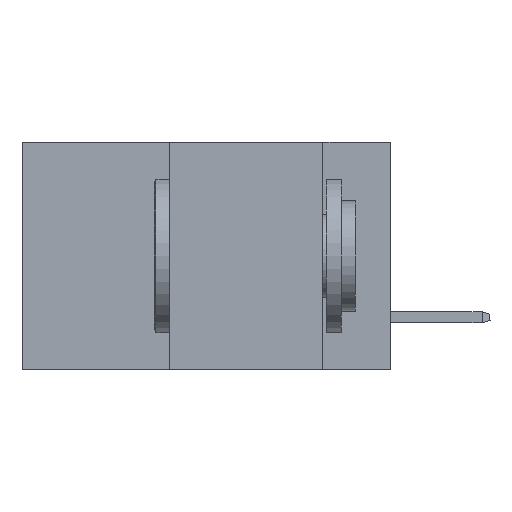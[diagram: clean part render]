
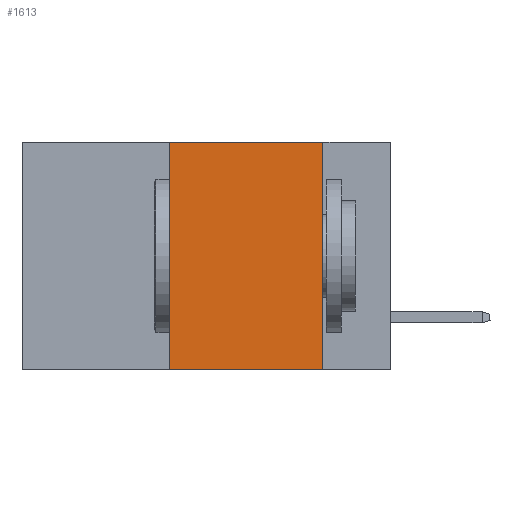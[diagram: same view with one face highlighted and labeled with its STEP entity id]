
A CAD part, left-side view. The second image highlights one B-rep face of the part: STEP entity #1613.
In plain terms, the highlighted planar face has unit normal (-1, 0, 0).
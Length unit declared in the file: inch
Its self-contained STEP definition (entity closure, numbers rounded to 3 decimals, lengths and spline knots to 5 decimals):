
#609 = EDGE_LOOP ( 'NONE', ( #4882, #5070, #9992, #18056 ) ) ;
#1401 = DIRECTION ( 'NONE',  ( 0., 0., 1. ) ) ;
#1613 = ADVANCED_FACE ( 'NONE', ( #8489 ), #11066, .F. ) ;
#1796 = AXIS2_PLACEMENT_3D ( 'NONE', #4630, #11137, #4764 ) ;
#3876 = VERTEX_POINT ( 'NONE', #20409 ) ;
#4294 = CARTESIAN_POINT ( 'NONE',  ( 0., 0.11, -0.37 ) ) ;
#4630 = CARTESIAN_POINT ( 'NONE',  ( 0., 0.6, 0. ) ) ;
#4764 = DIRECTION ( 'NONE',  ( 0., 0., -1. ) ) ;
#4882 = ORIENTED_EDGE ( 'NONE', *, *, #19398, .F. ) ;
#5070 = ORIENTED_EDGE ( 'NONE', *, *, #13907, .F. ) ;
#5511 = DIRECTION ( 'NONE',  ( 0., -1., 0. ) ) ;
#6402 = VERTEX_POINT ( 'NONE', #14338 ) ;
#6741 = LINE ( 'NONE', #7772, #8992 ) ;
#7194 = VERTEX_POINT ( 'NONE', #10038 ) ;
#7772 = CARTESIAN_POINT ( 'NONE',  ( 0., 0.6, 0. ) ) ;
#8489 = FACE_OUTER_BOUND ( 'NONE', #609, .T. ) ;
#8992 = VECTOR ( 'NONE', #10827, 39.37008 ) ;
#9992 = ORIENTED_EDGE ( 'NONE', *, *, #19097, .F. ) ;
#10038 = CARTESIAN_POINT ( 'NONE',  ( 0., 0.36, 0. ) ) ;
#10827 = DIRECTION ( 'NONE',  ( 0., -1., 0. ) ) ;
#11066 = PLANE ( 'NONE',  #1796 ) ;
#11137 = DIRECTION ( 'NONE',  ( 1., 0., 0. ) ) ;
#11855 = EDGE_CURVE ( 'NONE', #6402, #17777, #16353, .T. ) ;
#12032 = LINE ( 'NONE', #14416, #18344 ) ;
#12277 = LINE ( 'NONE', #13844, #14544 ) ;
#12330 = VECTOR ( 'NONE', #5511, 39.37008 ) ;
#13844 = CARTESIAN_POINT ( 'NONE',  ( 0., 0.11, 0. ) ) ;
#13907 = EDGE_CURVE ( 'NONE', #7194, #3876, #6741, .T. ) ;
#14338 = CARTESIAN_POINT ( 'NONE',  ( 0., 0.36, -0.37 ) ) ;
#14416 = CARTESIAN_POINT ( 'NONE',  ( 0., 0.36, 0. ) ) ;
#14544 = VECTOR ( 'NONE', #15391, 39.37008 ) ;
#15391 = DIRECTION ( 'NONE',  ( 0., 0., -1. ) ) ;
#16353 = LINE ( 'NONE', #20042, #12330 ) ;
#17777 = VERTEX_POINT ( 'NONE', #4294 ) ;
#18056 = ORIENTED_EDGE ( 'NONE', *, *, #11855, .T. ) ;
#18344 = VECTOR ( 'NONE', #1401, 39.37008 ) ;
#19097 = EDGE_CURVE ( 'NONE', #6402, #7194, #12032, .T. ) ;
#19398 = EDGE_CURVE ( 'NONE', #3876, #17777, #12277, .T. ) ;
#20042 = CARTESIAN_POINT ( 'NONE',  ( 0., 0.6, -0.37 ) ) ;
#20409 = CARTESIAN_POINT ( 'NONE',  ( 0., 0.11, 0. ) ) ;
